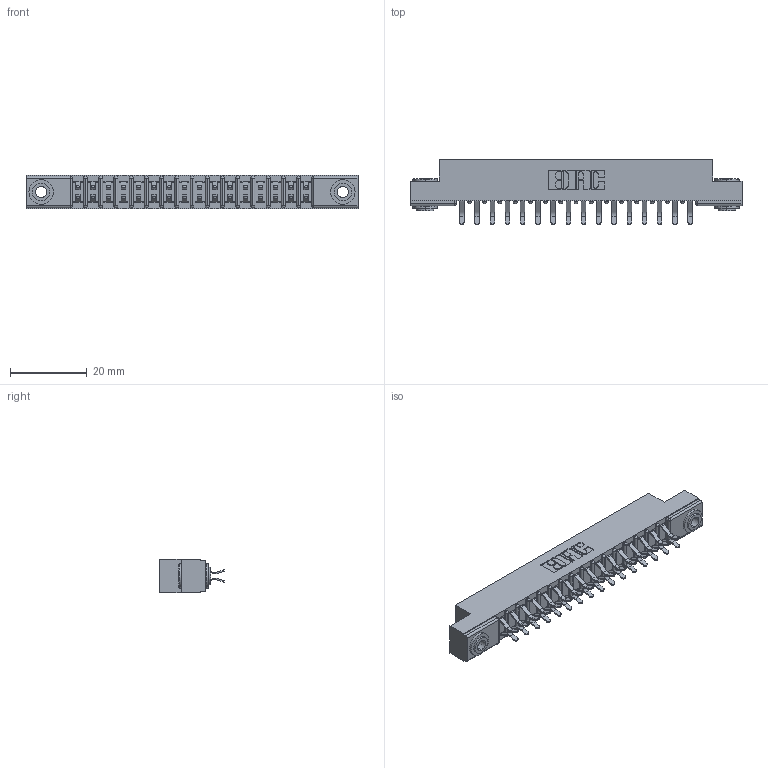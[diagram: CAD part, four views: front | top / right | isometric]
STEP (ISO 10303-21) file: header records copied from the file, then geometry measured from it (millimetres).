
FILE_DESCRIPTION (( 'STEP AP203' ), '1' );
FILE_NAME ('307-032-456-203.STEP', '2020-09-29T11:27:51', ( '' ), ( '' ), 'SwSTEP 2.0', 'SolidWorks 2020', '' );
FILE_SCHEMA (( 'CONFIG_CONTROL_DESIGN' ));
Length unit declared in the file: inch
Products named in the file (4): 307 Part_.156 Dia Mounting Holes; 307-290-001_556; 307-032-456-203; 345-250-002_345-250-002-102
Assembly tree (35 placements, depth 2):
  307-032-456-203
    307 Part_.156 Dia Mounting Holes
    307-290-001_556  x32
    345-250-002_345-250-002-102  x2
Bounding box: 86.41 x 16.97 x 8.71 mm (x, y, z)
Volume: 5648.4 mm3; surface area: 9878.8 mm2
Topology: 35 solids, 35 shells, 1787 faces, 4979 edges, 3226 vertices
Faces by surface type: plane 1150, cylinder 595, sphere 34, cone 8
Entity records: 18603 total; most frequent: CARTESIAN_POINT 3033, DIRECTION 2997, ORIENTED_EDGE 2994, EDGE_CURVE 1497, LINE 1129, VECTOR 1129, VERTEX_POINT 970, AXIS2_PLACEMENT_3D 934
